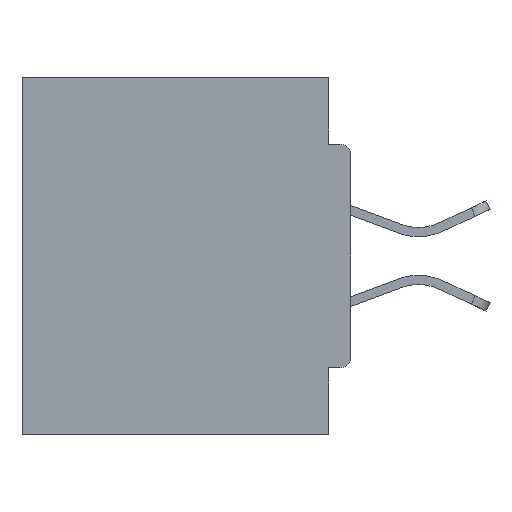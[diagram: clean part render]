
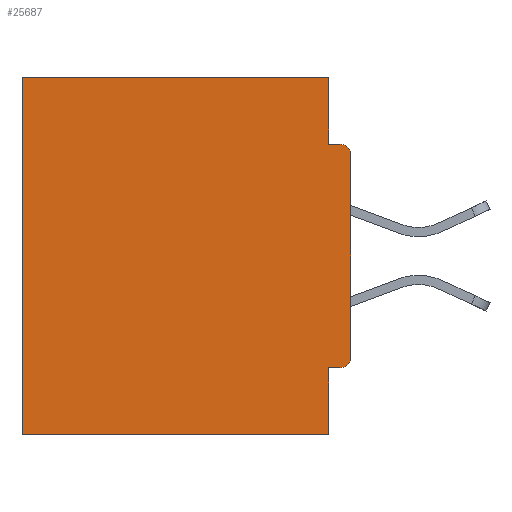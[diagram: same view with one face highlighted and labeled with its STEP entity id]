
A CAD part, left-side view. The second image highlights one B-rep face of the part: STEP entity #25687.
In plain terms, the highlighted planar face has unit normal (-1, 0, 0).
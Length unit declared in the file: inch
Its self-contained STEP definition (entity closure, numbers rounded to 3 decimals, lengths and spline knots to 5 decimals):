
#62 = CARTESIAN_POINT ( 'NONE',  ( 0.298, 0., -0.1085 ) ) ;
#141 = CARTESIAN_POINT ( 'NONE',  ( 0.298, 0.46, -0.5 ) ) ;
#142 = EDGE_CURVE ( 'NONE', #19413, #34397, #34042, .T. ) ;
#262 = LINE ( 'NONE', #30924, #33901 ) ;
#538 = EDGE_CURVE ( 'NONE', #8343, #23334, #34425, .T. ) ;
#562 = VECTOR ( 'NONE', #12898, 39.37008 ) ;
#571 = LINE ( 'NONE', #29517, #16116 ) ;
#1081 = DIRECTION ( 'NONE',  ( 0., 0., -1. ) ) ;
#1180 = VERTEX_POINT ( 'NONE', #11008 ) ;
#1301 = CARTESIAN_POINT ( 'NONE',  ( 0.298, 0., -0.4065 ) ) ;
#1895 = DIRECTION ( 'NONE',  ( -1., 0., 0. ) ) ;
#2771 = ORIENTED_EDGE ( 'NONE', *, *, #26138, .T. ) ;
#3373 = CARTESIAN_POINT ( 'NONE',  ( 0.298, 0.46, 0. ) ) ;
#3513 = VECTOR ( 'NONE', #25401, 39.37008 ) ;
#4736 = DIRECTION ( 'NONE',  ( 0., 0., -1. ) ) ;
#5084 = CARTESIAN_POINT ( 'NONE',  ( 0.298, 0.031, 0. ) ) ;
#5232 = VERTEX_POINT ( 'NONE', #17488 ) ;
#5280 = EDGE_CURVE ( 'NONE', #19413, #26836, #262, .T. ) ;
#6215 = VERTEX_POINT ( 'NONE', #29824 ) ;
#6342 = EDGE_CURVE ( 'NONE', #6215, #24206, #7306, .T. ) ;
#6465 = VECTOR ( 'NONE', #28717, 39.37008 ) ;
#7306 = LINE ( 'NONE', #26226, #6465 ) ;
#8246 = ORIENTED_EDGE ( 'NONE', *, *, #32245, .F. ) ;
#8343 = VERTEX_POINT ( 'NONE', #62 ) ;
#8444 = AXIS2_PLACEMENT_3D ( 'NONE', #19645, #25178, #1081 ) ;
#8889 = LINE ( 'NONE', #11827, #15147 ) ;
#9305 = EDGE_LOOP ( 'NONE', ( #10855, #26342, #22728, #10143, #26846, #28266, #8246, #21200, #2771, #30719 ) ) ;
#9420 = VERTEX_POINT ( 'NONE', #12896 ) ;
#10143 = ORIENTED_EDGE ( 'NONE', *, *, #142, .T. ) ;
#10291 = CARTESIAN_POINT ( 'NONE',  ( 0.298, 0., 0. ) ) ;
#10855 = ORIENTED_EDGE ( 'NONE', *, *, #538, .T. ) ;
#11008 = CARTESIAN_POINT ( 'NONE',  ( 0.298, 0.015, -0.4065 ) ) ;
#11258 = EDGE_CURVE ( 'NONE', #1180, #9420, #18619, .T. ) ;
#11758 = DIRECTION ( 'NONE',  ( 0., 0., -1. ) ) ;
#11827 = CARTESIAN_POINT ( 'NONE',  ( 0.298, 0.031, -0.5 ) ) ;
#12691 = CARTESIAN_POINT ( 'NONE',  ( 0.298, 0.031, -0.0935 ) ) ;
#12896 = CARTESIAN_POINT ( 'NONE',  ( 0.298, 0.031, -0.4065 ) ) ;
#12898 = DIRECTION ( 'NONE',  ( 0., -1., 0. ) ) ;
#14358 = EDGE_CURVE ( 'NONE', #8343, #5232, #571, .T. ) ;
#15147 = VECTOR ( 'NONE', #16991, 39.37008 ) ;
#15392 = AXIS2_PLACEMENT_3D ( 'NONE', #30628, #22727, #19912 ) ;
#16116 = VECTOR ( 'NONE', #18642, 39.37008 ) ;
#16991 = DIRECTION ( 'NONE',  ( 0., 0., -1. ) ) ;
#17488 = CARTESIAN_POINT ( 'NONE',  ( 0.298, 0., -0.3915 ) ) ;
#17715 = EDGE_CURVE ( 'NONE', #34397, #24206, #31488, .T. ) ;
#18619 = LINE ( 'NONE', #1301, #3513 ) ;
#18642 = DIRECTION ( 'NONE',  ( 0., 0., -1. ) ) ;
#18912 = CIRCLE ( 'NONE', #15392, 0.015 ) ;
#19304 = VECTOR ( 'NONE', #23957, 39.37008 ) ;
#19413 = VERTEX_POINT ( 'NONE', #5084 ) ;
#19645 = CARTESIAN_POINT ( 'NONE',  ( 0.298, 0., 0. ) ) ;
#19912 = DIRECTION ( 'NONE',  ( 0., 0., -1. ) ) ;
#21200 = ORIENTED_EDGE ( 'NONE', *, *, #11258, .F. ) ;
#21842 = AXIS2_PLACEMENT_3D ( 'NONE', #23884, #1895, #4736 ) ;
#22120 = EDGE_CURVE ( 'NONE', #26836, #23334, #30034, .T. ) ;
#22727 = DIRECTION ( 'NONE',  ( -1., 0., 0. ) ) ;
#22728 = ORIENTED_EDGE ( 'NONE', *, *, #5280, .F. ) ;
#23334 = VERTEX_POINT ( 'NONE', #31010 ) ;
#23884 = CARTESIAN_POINT ( 'NONE',  ( 0.298, 0.015, -0.1085 ) ) ;
#23957 = DIRECTION ( 'NONE',  ( 0., 1., 0. ) ) ;
#24206 = VERTEX_POINT ( 'NONE', #141 ) ;
#25178 = DIRECTION ( 'NONE',  ( 1., 0., 0. ) ) ;
#25330 = DIRECTION ( 'NONE',  ( 0., 0., -1. ) ) ;
#25401 = DIRECTION ( 'NONE',  ( 0., 1., 0. ) ) ;
#25687 = ADVANCED_FACE ( 'NONE', ( #33244 ), #32966, .F. ) ;
#26138 = EDGE_CURVE ( 'NONE', #1180, #5232, #18912, .T. ) ;
#26226 = CARTESIAN_POINT ( 'NONE',  ( 0.298, 0., -0.5 ) ) ;
#26342 = ORIENTED_EDGE ( 'NONE', *, *, #22120, .F. ) ;
#26836 = VERTEX_POINT ( 'NONE', #12691 ) ;
#26846 = ORIENTED_EDGE ( 'NONE', *, *, #17715, .T. ) ;
#28266 = ORIENTED_EDGE ( 'NONE', *, *, #6342, .F. ) ;
#28717 = DIRECTION ( 'NONE',  ( 0., 1., 0. ) ) ;
#29517 = CARTESIAN_POINT ( 'NONE',  ( 0.298, 0., 0. ) ) ;
#29824 = CARTESIAN_POINT ( 'NONE',  ( 0.298, 0.031, -0.5 ) ) ;
#30034 = LINE ( 'NONE', #34314, #562 ) ;
#30628 = CARTESIAN_POINT ( 'NONE',  ( 0.298, 0.015, -0.3915 ) ) ;
#30646 = VECTOR ( 'NONE', #25330, 39.37008 ) ;
#30719 = ORIENTED_EDGE ( 'NONE', *, *, #14358, .F. ) ;
#30924 = CARTESIAN_POINT ( 'NONE',  ( 0.298, 0.031, -0.5 ) ) ;
#31010 = CARTESIAN_POINT ( 'NONE',  ( 0.298, 0.015, -0.0935 ) ) ;
#31488 = LINE ( 'NONE', #3373, #30646 ) ;
#31564 = CARTESIAN_POINT ( 'NONE',  ( 0.298, 0.46, 0. ) ) ;
#32245 = EDGE_CURVE ( 'NONE', #9420, #6215, #8889, .T. ) ;
#32966 = PLANE ( 'NONE',  #8444 ) ;
#33244 = FACE_OUTER_BOUND ( 'NONE', #9305, .T. ) ;
#33901 = VECTOR ( 'NONE', #11758, 39.37008 ) ;
#34042 = LINE ( 'NONE', #10291, #19304 ) ;
#34314 = CARTESIAN_POINT ( 'NONE',  ( 0.298, 0., -0.0935 ) ) ;
#34397 = VERTEX_POINT ( 'NONE', #31564 ) ;
#34425 = CIRCLE ( 'NONE', #21842, 0.015 ) ;
